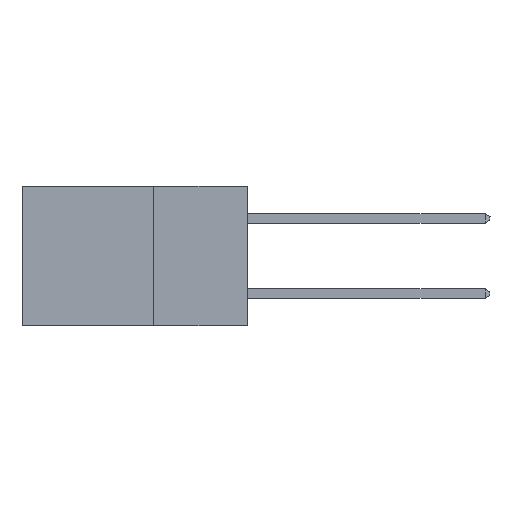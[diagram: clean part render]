
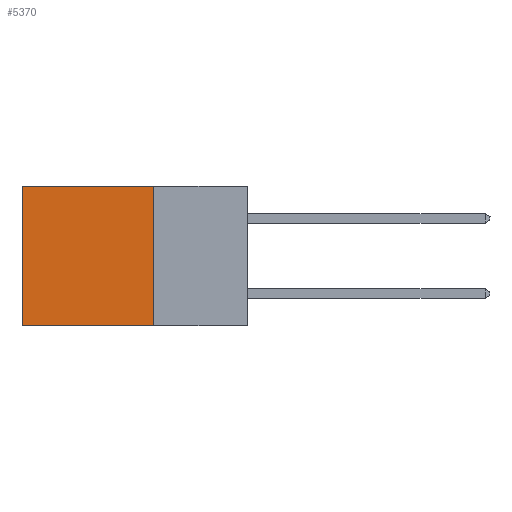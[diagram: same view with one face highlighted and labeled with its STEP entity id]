
A CAD part, left-side view. The second image highlights one B-rep face of the part: STEP entity #5370.
In plain terms, the highlighted planar face has unit normal (-1, 0, 0).
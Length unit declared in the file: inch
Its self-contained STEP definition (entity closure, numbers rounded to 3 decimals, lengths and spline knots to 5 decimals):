
#1031 = ORIENTED_EDGE ( 'NONE', *, *, #18094, .F. ) ;
#1300 = CARTESIAN_POINT ( 'NONE',  ( 0.2615, 0.25, 0. ) ) ;
#1943 = VECTOR ( 'NONE', #3900, 39.37008 ) ;
#2226 = CARTESIAN_POINT ( 'NONE',  ( 0.2615, 0.25, 0. ) ) ;
#3442 = VECTOR ( 'NONE', #4767, 39.37008 ) ;
#3654 = ORIENTED_EDGE ( 'NONE', *, *, #10318, .T. ) ;
#3900 = DIRECTION ( 'NONE',  ( 0., 0., -1. ) ) ;
#4767 = DIRECTION ( 'NONE',  ( 0., 0., -1. ) ) ;
#5370 = ADVANCED_FACE ( 'NONE', ( #7078 ), #18990, .F. ) ;
#5453 = EDGE_CURVE ( 'NONE', #16391, #12024, #9042, .T. ) ;
#5807 = EDGE_CURVE ( 'NONE', #13453, #17328, #6971, .T. ) ;
#5984 = ORIENTED_EDGE ( 'NONE', *, *, #5807, .T. ) ;
#6971 = LINE ( 'NONE', #1300, #9076 ) ;
#7078 = FACE_OUTER_BOUND ( 'NONE', #15096, .T. ) ;
#7284 = DIRECTION ( 'NONE',  ( 1., 0., 0. ) ) ;
#7690 = LINE ( 'NONE', #15256, #3442 ) ;
#7734 = ORIENTED_EDGE ( 'NONE', *, *, #5453, .F. ) ;
#9042 = LINE ( 'NONE', #18196, #11507 ) ;
#9076 = VECTOR ( 'NONE', #11303, 39.37008 ) ;
#9546 = CARTESIAN_POINT ( 'NONE',  ( 0.2615, 0.6, -0.37 ) ) ;
#10318 = EDGE_CURVE ( 'NONE', #17328, #12024, #7690, .T. ) ;
#11303 = DIRECTION ( 'NONE',  ( 0., 1., 0. ) ) ;
#11342 = LINE ( 'NONE', #15564, #1943 ) ;
#11507 = VECTOR ( 'NONE', #17985, 39.37008 ) ;
#12024 = VERTEX_POINT ( 'NONE', #9546 ) ;
#13453 = VERTEX_POINT ( 'NONE', #2226 ) ;
#14780 = CARTESIAN_POINT ( 'NONE',  ( 0.2615, 0.25, -0.37 ) ) ;
#15096 = EDGE_LOOP ( 'NONE', ( #3654, #7734, #1031, #5984 ) ) ;
#15256 = CARTESIAN_POINT ( 'NONE',  ( 0.2615, 0.6, -0.37 ) ) ;
#15564 = CARTESIAN_POINT ( 'NONE',  ( 0.2615, 0.25, -0.37 ) ) ;
#16391 = VERTEX_POINT ( 'NONE', #14780 ) ;
#17328 = VERTEX_POINT ( 'NONE', #19147 ) ;
#17985 = DIRECTION ( 'NONE',  ( 0., 1., 0. ) ) ;
#18094 = EDGE_CURVE ( 'NONE', #13453, #16391, #11342, .T. ) ;
#18196 = CARTESIAN_POINT ( 'NONE',  ( 0.2615, 0.25, -0.37 ) ) ;
#18990 = PLANE ( 'NONE',  #19047 ) ;
#19047 = AXIS2_PLACEMENT_3D ( 'NONE', #19183, #7284, #19263 ) ;
#19147 = CARTESIAN_POINT ( 'NONE',  ( 0.2615, 0.6, 0. ) ) ;
#19183 = CARTESIAN_POINT ( 'NONE',  ( 0.2615, 0.25, -0.37 ) ) ;
#19263 = DIRECTION ( 'NONE',  ( 0., 0., -1. ) ) ;
